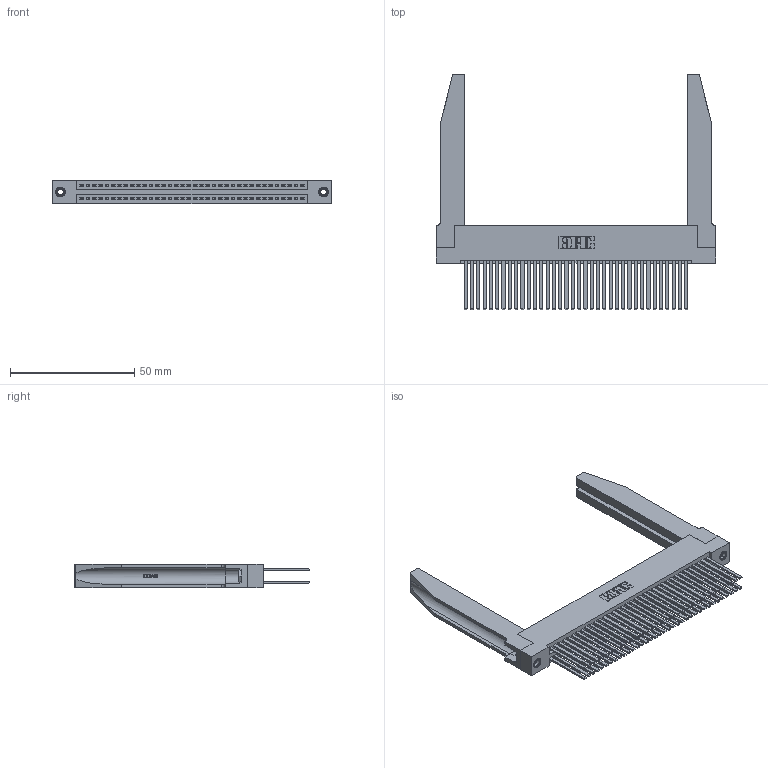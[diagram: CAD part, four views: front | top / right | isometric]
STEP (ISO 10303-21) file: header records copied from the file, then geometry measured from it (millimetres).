
FILE_DESCRIPTION (( 'STEP AP203' ), '1' );
FILE_NAME ('345-072-544-278.STEP', '2019-10-31T04:01:30', ( '' ), ( '' ), 'SwSTEP 2.0', 'SolidWorks 2016', '' );
FILE_SCHEMA (( 'CONFIG_CONTROL_DESIGN' ));
Length unit declared in the file: inch
Products named in the file (5): 345 Part_Flush Mounting Lugs - 0.156 Dia-TH; 345-220-078_345-220-078; 345-292-001_345-293-144; 345-250-001_345-250-001-102; 345-072-544-278
Assembly tree (77 placements, depth 2):
  345-072-544-278
    345 Part_Flush Mounting Lugs - 0.156 Dia-TH
    345-292-001_345-293-144  x72
    345-250-001_345-250-001-102  x2
    345-220-078_345-220-078  x2
Bounding box: 112.67 x 94.92 x 9.4 mm (x, y, z)
Volume: 19669.3 mm3; surface area: 27269 mm2
Topology: 77 solids, 77 shells, 3528 faces, 10381 edges, 6814 vertices
Faces by surface type: plane 2310, cylinder 1166, bspline 36, cone 12, torus 4
Entity records: 33610 total; most frequent: CARTESIAN_POINT 6555, ORIENTED_EDGE 5386, DIRECTION 4779, EDGE_CURVE 2693, VECTOR 2327, LINE 2327, VERTEX_POINT 1788, AXIS2_PLACEMENT_3D 1226
